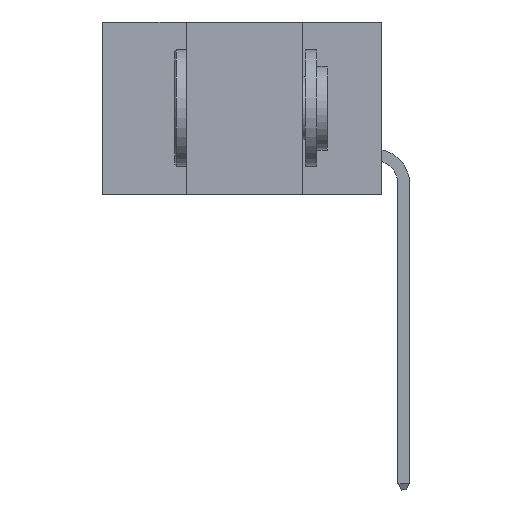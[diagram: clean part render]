
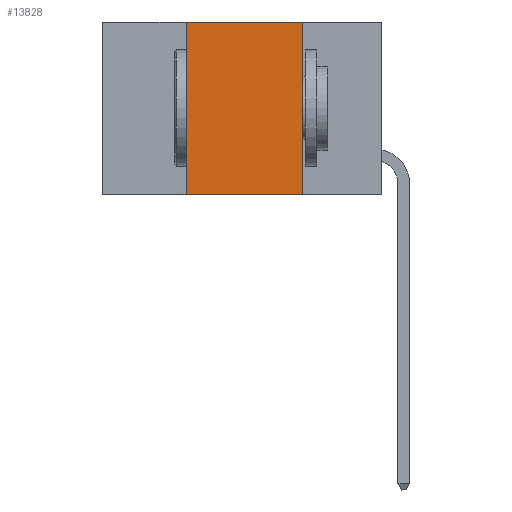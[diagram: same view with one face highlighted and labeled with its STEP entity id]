
A CAD part, left-side view. The second image highlights one B-rep face of the part: STEP entity #13828.
In plain terms, the highlighted planar face has unit normal (-1, 0, 0).
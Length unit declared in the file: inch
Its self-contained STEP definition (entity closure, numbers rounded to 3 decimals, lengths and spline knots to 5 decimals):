
#861 = LINE ( 'NONE', #13064, #10753 ) ;
#1550 = VERTEX_POINT ( 'NONE', #6289 ) ;
#4009 = DIRECTION ( 'NONE',  ( 0., 0., -1. ) ) ;
#4857 = CARTESIAN_POINT ( 'NONE',  ( 0., 0.6, -0.37 ) ) ;
#5756 = DIRECTION ( 'NONE',  ( 1., 0., 0. ) ) ;
#6289 = CARTESIAN_POINT ( 'NONE',  ( 0., 0.17, 0. ) ) ;
#6500 = ORIENTED_EDGE ( 'NONE', *, *, #28618, .F. ) ;
#6838 = VECTOR ( 'NONE', #24870, 39.37008 ) ;
#7529 = VERTEX_POINT ( 'NONE', #23433 ) ;
#7909 = EDGE_CURVE ( 'NONE', #7529, #16028, #34731, .T. ) ;
#10753 = VECTOR ( 'NONE', #37321, 39.37008 ) ;
#13064 = CARTESIAN_POINT ( 'NONE',  ( 0., 0.6, 0. ) ) ;
#13828 = ADVANCED_FACE ( 'NONE', ( #21993 ), #13912, .F. ) ;
#13912 = PLANE ( 'NONE',  #38215 ) ;
#14872 = CARTESIAN_POINT ( 'NONE',  ( 0., 0.17, -0.37 ) ) ;
#15448 = VERTEX_POINT ( 'NONE', #46645 ) ;
#16028 = VERTEX_POINT ( 'NONE', #14872 ) ;
#18635 = EDGE_CURVE ( 'NONE', #1550, #16028, #45243, .T. ) ;
#19801 = LINE ( 'NONE', #49827, #28221 ) ;
#21122 = DIRECTION ( 'NONE',  ( 0., 0., 1. ) ) ;
#21993 = FACE_OUTER_BOUND ( 'NONE', #48910, .T. ) ;
#23433 = CARTESIAN_POINT ( 'NONE',  ( 0., 0.42, -0.37 ) ) ;
#24870 = DIRECTION ( 'NONE',  ( 0., -1., 0. ) ) ;
#28221 = VECTOR ( 'NONE', #21122, 39.37008 ) ;
#28618 = EDGE_CURVE ( 'NONE', #15448, #1550, #861, .T. ) ;
#28799 = EDGE_CURVE ( 'NONE', #7529, #15448, #19801, .T. ) ;
#30245 = CARTESIAN_POINT ( 'NONE',  ( 0., 0.17, 0. ) ) ;
#31384 = ORIENTED_EDGE ( 'NONE', *, *, #28799, .F. ) ;
#31944 = ORIENTED_EDGE ( 'NONE', *, *, #7909, .T. ) ;
#32328 = VECTOR ( 'NONE', #4009, 39.37008 ) ;
#33666 = ORIENTED_EDGE ( 'NONE', *, *, #18635, .F. ) ;
#34731 = LINE ( 'NONE', #4857, #6838 ) ;
#36649 = CARTESIAN_POINT ( 'NONE',  ( 0., 0.6, 0. ) ) ;
#37321 = DIRECTION ( 'NONE',  ( 0., -1., 0. ) ) ;
#38215 = AXIS2_PLACEMENT_3D ( 'NONE', #36649, #5756, #48762 ) ;
#45243 = LINE ( 'NONE', #30245, #32328 ) ;
#46645 = CARTESIAN_POINT ( 'NONE',  ( 0., 0.42, 0. ) ) ;
#48762 = DIRECTION ( 'NONE',  ( 0., 0., -1. ) ) ;
#48910 = EDGE_LOOP ( 'NONE', ( #33666, #6500, #31384, #31944 ) ) ;
#49827 = CARTESIAN_POINT ( 'NONE',  ( 0., 0.42, 0. ) ) ;
